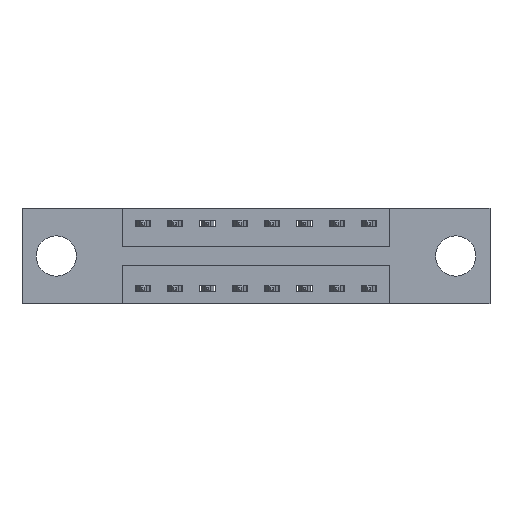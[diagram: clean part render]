
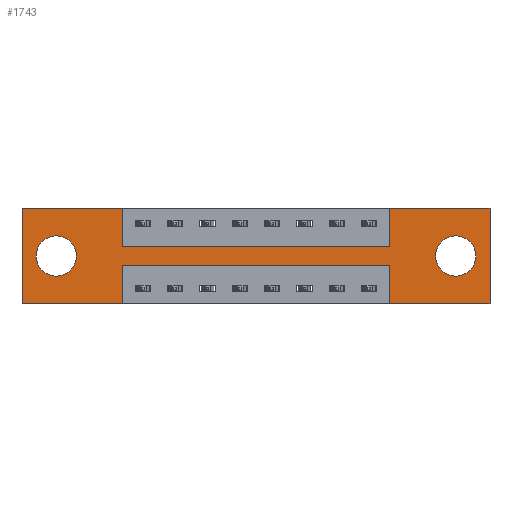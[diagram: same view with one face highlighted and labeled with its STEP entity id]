
A CAD part, front view. The second image highlights one B-rep face of the part: STEP entity #1743.
In plain terms, the highlighted planar face has unit normal (0, -1, 0).
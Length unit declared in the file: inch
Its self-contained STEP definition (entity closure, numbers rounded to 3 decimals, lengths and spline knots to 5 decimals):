
#112 = CARTESIAN_POINT ( 'NONE',  ( 1.4225, 0., 0. ) ) ;
#200 = VECTOR ( 'NONE', #9709, 39.37008 ) ;
#206 = ORIENTED_EDGE ( 'NONE', *, *, #6975, .F. ) ;
#321 = CARTESIAN_POINT ( 'NONE',  ( 0., 0., 0. ) ) ;
#332 = FACE_BOUND ( 'NONE', #2129, .T. ) ;
#373 = VERTEX_POINT ( 'NONE', #10137 ) ;
#382 = PLANE ( 'NONE',  #7027 ) ;
#436 = FACE_OUTER_BOUND ( 'NONE', #8630, .T. ) ;
#615 = EDGE_CURVE ( 'NONE', #1012, #9440, #9517, .T. ) ;
#698 = DIRECTION ( 'NONE',  ( 1., 0., 0. ) ) ;
#814 = ORIENTED_EDGE ( 'NONE', *, *, #615, .F. ) ;
#889 = DIRECTION ( 'NONE',  ( -1., 0., 0. ) ) ;
#936 = ORIENTED_EDGE ( 'NONE', *, *, #5097, .T. ) ;
#983 = CIRCLE ( 'NONE', #4467, 0.078 ) ;
#1012 = VERTEX_POINT ( 'NONE', #8570 ) ;
#1128 = AXIS2_PLACEMENT_3D ( 'NONE', #7629, #1554, #7058 ) ;
#1171 = EDGE_CURVE ( 'NONE', #3904, #6323, #5611, .T. ) ;
#1223 = LINE ( 'NONE', #7734, #9529 ) ;
#1234 = CARTESIAN_POINT ( 'NONE',  ( 1.81, 0., 0. ) ) ;
#1289 = ORIENTED_EDGE ( 'NONE', *, *, #1171, .F. ) ;
#1308 = DIRECTION ( 'NONE',  ( 0., 0., 1. ) ) ;
#1554 = DIRECTION ( 'NONE',  ( 0., 1., 0. ) ) ;
#1563 = EDGE_CURVE ( 'NONE', #7716, #8273, #3707, .T. ) ;
#1653 = CARTESIAN_POINT ( 'NONE',  ( 1.81, 0., -0.37 ) ) ;
#1743 = ADVANCED_FACE ( 'NONE', ( #332, #6601, #436 ), #382, .T. ) ;
#1836 = DIRECTION ( 'NONE',  ( 0., 0., -1. ) ) ;
#1846 = AXIS2_PLACEMENT_3D ( 'NONE', #10149, #6109, #1308 ) ;
#1887 = CARTESIAN_POINT ( 'NONE',  ( 1.81, 0., 0. ) ) ;
#1895 = EDGE_CURVE ( 'NONE', #4894, #4842, #983, .T. ) ;
#1976 = LINE ( 'NONE', #1887, #8214 ) ;
#2050 = VERTEX_POINT ( 'NONE', #4243 ) ;
#2129 = EDGE_LOOP ( 'NONE', ( #8055, #8114 ) ) ;
#2205 = CARTESIAN_POINT ( 'NONE',  ( 1.6775, 0., -0.263 ) ) ;
#2235 = DIRECTION ( 'NONE',  ( 0., 0., -1. ) ) ;
#2417 = CARTESIAN_POINT ( 'NONE',  ( 0., 0., 0. ) ) ;
#2439 = CARTESIAN_POINT ( 'NONE',  ( 0., 0., 0. ) ) ;
#2569 = DIRECTION ( 'NONE',  ( 1., 0., 0. ) ) ;
#2634 = CARTESIAN_POINT ( 'NONE',  ( 0., 0., -0.37 ) ) ;
#2875 = VECTOR ( 'NONE', #889, 39.37008 ) ;
#2906 = EDGE_CURVE ( 'NONE', #9912, #5374, #5189, .T. ) ;
#3069 = ORIENTED_EDGE ( 'NONE', *, *, #1895, .T. ) ;
#3085 = LINE ( 'NONE', #10248, #6941 ) ;
#3213 = VECTOR ( 'NONE', #8144, 39.37008 ) ;
#3224 = EDGE_CURVE ( 'NONE', #2050, #9912, #5714, .T. ) ;
#3422 = CARTESIAN_POINT ( 'NONE',  ( 0.1325, 0., -0.263 ) ) ;
#3502 = LINE ( 'NONE', #9997, #3623 ) ;
#3506 = CARTESIAN_POINT ( 'NONE',  ( 0.3875, 0., -0.15 ) ) ;
#3512 = CARTESIAN_POINT ( 'NONE',  ( 0.1325, 0., -0.107 ) ) ;
#3623 = VECTOR ( 'NONE', #3649, 39.37008 ) ;
#3649 = DIRECTION ( 'NONE',  ( 0., 0., 1. ) ) ;
#3703 = ORIENTED_EDGE ( 'NONE', *, *, #6094, .F. ) ;
#3707 = CIRCLE ( 'NONE', #4538, 0.078 ) ;
#3762 = CARTESIAN_POINT ( 'NONE',  ( 0.3875, 0., -0.22 ) ) ;
#3835 = DIRECTION ( 'NONE',  ( 0., 1., 0. ) ) ;
#3904 = VERTEX_POINT ( 'NONE', #2634 ) ;
#3942 = LINE ( 'NONE', #9459, #2875 ) ;
#4147 = ORIENTED_EDGE ( 'NONE', *, *, #2906, .F. ) ;
#4178 = EDGE_CURVE ( 'NONE', #6323, #7251, #7920, .T. ) ;
#4243 = CARTESIAN_POINT ( 'NONE',  ( 1.4225, 0., -0.15 ) ) ;
#4400 = DIRECTION ( 'NONE',  ( -1., 0., 0. ) ) ;
#4426 = CARTESIAN_POINT ( 'NONE',  ( 1.6775, 0., -0.185 ) ) ;
#4467 = AXIS2_PLACEMENT_3D ( 'NONE', #9987, #3835, #7889 ) ;
#4538 = AXIS2_PLACEMENT_3D ( 'NONE', #4426, #5800, #1836 ) ;
#4667 = CARTESIAN_POINT ( 'NONE',  ( 0.3875, 0., -0.37 ) ) ;
#4726 = ORIENTED_EDGE ( 'NONE', *, *, #3224, .F. ) ;
#4842 = VERTEX_POINT ( 'NONE', #3422 ) ;
#4894 = VERTEX_POINT ( 'NONE', #3512 ) ;
#4956 = CARTESIAN_POINT ( 'NONE',  ( 0.3875, 0., 0. ) ) ;
#5097 = EDGE_CURVE ( 'NONE', #4842, #4894, #9818, .T. ) ;
#5189 = LINE ( 'NONE', #321, #5496 ) ;
#5351 = CARTESIAN_POINT ( 'NONE',  ( 1.4225, 0., -0.37 ) ) ;
#5374 = VERTEX_POINT ( 'NONE', #1234 ) ;
#5397 = DIRECTION ( 'NONE',  ( -1., 0., 0. ) ) ;
#5496 = VECTOR ( 'NONE', #6855, 39.37008 ) ;
#5530 = CARTESIAN_POINT ( 'NONE',  ( 0.3875, 0., -0.37 ) ) ;
#5611 = LINE ( 'NONE', #2417, #3213 ) ;
#5616 = CARTESIAN_POINT ( 'NONE',  ( 1.6775, 0., -0.107 ) ) ;
#5691 = CARTESIAN_POINT ( 'NONE',  ( 0.3875, 0., 0. ) ) ;
#5714 = LINE ( 'NONE', #112, #200 ) ;
#5783 = ORIENTED_EDGE ( 'NONE', *, *, #6702, .F. ) ;
#5800 = DIRECTION ( 'NONE',  ( 0., 1., 0. ) ) ;
#6094 = EDGE_CURVE ( 'NONE', #9302, #373, #3502, .T. ) ;
#6109 = DIRECTION ( 'NONE',  ( 0., 1., 0. ) ) ;
#6214 = EDGE_CURVE ( 'NONE', #6997, #2050, #3085, .T. ) ;
#6323 = VERTEX_POINT ( 'NONE', #2439 ) ;
#6473 = EDGE_LOOP ( 'NONE', ( #3069, #936 ) ) ;
#6499 = EDGE_CURVE ( 'NONE', #8273, #7716, #10104, .T. ) ;
#6601 = FACE_BOUND ( 'NONE', #6473, .T. ) ;
#6611 = DIRECTION ( 'NONE',  ( 0., 0., -1. ) ) ;
#6659 = ORIENTED_EDGE ( 'NONE', *, *, #8538, .F. ) ;
#6702 = EDGE_CURVE ( 'NONE', #373, #1012, #8342, .T. ) ;
#6855 = DIRECTION ( 'NONE',  ( 1., 0., 0. ) ) ;
#6901 = ORIENTED_EDGE ( 'NONE', *, *, #9203, .F. ) ;
#6941 = VECTOR ( 'NONE', #698, 39.37008 ) ;
#6975 = EDGE_CURVE ( 'NONE', #7251, #6997, #9642, .T. ) ;
#6997 = VERTEX_POINT ( 'NONE', #3506 ) ;
#7027 = AXIS2_PLACEMENT_3D ( 'NONE', #8311, #9110, #9776 ) ;
#7058 = DIRECTION ( 'NONE',  ( 0., 0., -1. ) ) ;
#7114 = VECTOR ( 'NONE', #5397, 39.37008 ) ;
#7121 = VECTOR ( 'NONE', #8075, 39.37008 ) ;
#7136 = CARTESIAN_POINT ( 'NONE',  ( 0., 0., 0. ) ) ;
#7251 = VERTEX_POINT ( 'NONE', #5691 ) ;
#7629 = CARTESIAN_POINT ( 'NONE',  ( 1.6775, 0., -0.185 ) ) ;
#7716 = VERTEX_POINT ( 'NONE', #5616 ) ;
#7734 = CARTESIAN_POINT ( 'NONE',  ( 0., 0., -0.37 ) ) ;
#7842 = ORIENTED_EDGE ( 'NONE', *, *, #4178, .F. ) ;
#7889 = DIRECTION ( 'NONE',  ( 0., 0., 1. ) ) ;
#7920 = LINE ( 'NONE', #7136, #9989 ) ;
#8055 = ORIENTED_EDGE ( 'NONE', *, *, #1563, .T. ) ;
#8075 = DIRECTION ( 'NONE',  ( 0., 0., -1. ) ) ;
#8114 = ORIENTED_EDGE ( 'NONE', *, *, #6499, .T. ) ;
#8144 = DIRECTION ( 'NONE',  ( 0., 0., 1. ) ) ;
#8181 = VECTOR ( 'NONE', #2235, 39.37008 ) ;
#8214 = VECTOR ( 'NONE', #6611, 39.37008 ) ;
#8273 = VERTEX_POINT ( 'NONE', #2205 ) ;
#8306 = ORIENTED_EDGE ( 'NONE', *, *, #6214, .F. ) ;
#8311 = CARTESIAN_POINT ( 'NONE',  ( 0., 0., -0.37 ) ) ;
#8342 = LINE ( 'NONE', #3762, #7114 ) ;
#8370 = CARTESIAN_POINT ( 'NONE',  ( 1.4225, 0., 0. ) ) ;
#8538 = EDGE_CURVE ( 'NONE', #5374, #9233, #1976, .T. ) ;
#8570 = CARTESIAN_POINT ( 'NONE',  ( 0.3875, 0., -0.22 ) ) ;
#8630 = EDGE_LOOP ( 'NONE', ( #814, #5783, #3703, #10186, #6659, #4147, #4726, #8306, #206, #7842, #1289, #6901 ) ) ;
#9110 = DIRECTION ( 'NONE',  ( 0., -1., 0. ) ) ;
#9203 = EDGE_CURVE ( 'NONE', #9440, #3904, #3942, .T. ) ;
#9233 = VERTEX_POINT ( 'NONE', #1653 ) ;
#9302 = VERTEX_POINT ( 'NONE', #5351 ) ;
#9326 = EDGE_CURVE ( 'NONE', #9233, #9302, #1223, .T. ) ;
#9440 = VERTEX_POINT ( 'NONE', #4667 ) ;
#9459 = CARTESIAN_POINT ( 'NONE',  ( 0., 0., -0.37 ) ) ;
#9517 = LINE ( 'NONE', #5530, #8181 ) ;
#9529 = VECTOR ( 'NONE', #4400, 39.37008 ) ;
#9642 = LINE ( 'NONE', #4956, #7121 ) ;
#9709 = DIRECTION ( 'NONE',  ( 0., 0., 1. ) ) ;
#9776 = DIRECTION ( 'NONE',  ( 0., 0., -1. ) ) ;
#9818 = CIRCLE ( 'NONE', #1846, 0.078 ) ;
#9912 = VERTEX_POINT ( 'NONE', #8370 ) ;
#9987 = CARTESIAN_POINT ( 'NONE',  ( 0.1325, 0., -0.185 ) ) ;
#9989 = VECTOR ( 'NONE', #2569, 39.37008 ) ;
#9997 = CARTESIAN_POINT ( 'NONE',  ( 1.4225, 0., -0.37 ) ) ;
#10104 = CIRCLE ( 'NONE', #1128, 0.078 ) ;
#10137 = CARTESIAN_POINT ( 'NONE',  ( 1.4225, 0., -0.22 ) ) ;
#10149 = CARTESIAN_POINT ( 'NONE',  ( 0.1325, 0., -0.185 ) ) ;
#10186 = ORIENTED_EDGE ( 'NONE', *, *, #9326, .F. ) ;
#10248 = CARTESIAN_POINT ( 'NONE',  ( 0.3875, 0., -0.15 ) ) ;
